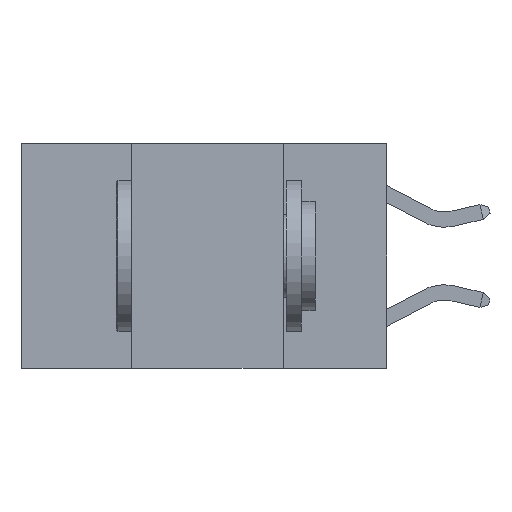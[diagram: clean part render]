
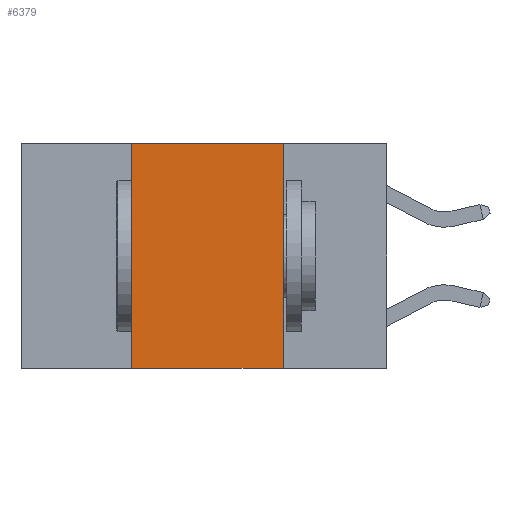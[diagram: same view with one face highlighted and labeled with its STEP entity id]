
A CAD part, left-side view. The second image highlights one B-rep face of the part: STEP entity #6379.
In plain terms, the highlighted planar face has unit normal (-1, 0, 0).
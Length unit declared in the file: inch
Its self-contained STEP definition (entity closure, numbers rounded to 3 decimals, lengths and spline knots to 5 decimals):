
#1246 = DIRECTION ( 'NONE',  ( 0., 0., 1. ) ) ;
#2895 = EDGE_CURVE ( 'NONE', #16272, #7749, #11159, .T. ) ;
#3063 = ORIENTED_EDGE ( 'NONE', *, *, #17406, .F. ) ;
#3518 = DIRECTION ( 'NONE',  ( 0., -1., 0. ) ) ;
#3544 = CARTESIAN_POINT ( 'NONE',  ( 0., 0.6, 0. ) ) ;
#4865 = VERTEX_POINT ( 'NONE', #10550 ) ;
#4994 = FACE_OUTER_BOUND ( 'NONE', #5014, .T. ) ;
#5014 = EDGE_LOOP ( 'NONE', ( #11372, #3063, #7511, #8008 ) ) ;
#5108 = EDGE_CURVE ( 'NONE', #4865, #9233, #6168, .T. ) ;
#5305 = CARTESIAN_POINT ( 'NONE',  ( 0., 0.17, 0. ) ) ;
#5511 = LINE ( 'NONE', #3544, #18115 ) ;
#5749 = VECTOR ( 'NONE', #3518, 39.37008 ) ;
#6168 = LINE ( 'NONE', #19264, #18697 ) ;
#6379 = ADVANCED_FACE ( 'NONE', ( #4994 ), #9672, .F. ) ;
#6440 = DIRECTION ( 'NONE',  ( 1., 0., 0. ) ) ;
#7029 = CARTESIAN_POINT ( 'NONE',  ( 0., 0.17, 0. ) ) ;
#7368 = EDGE_CURVE ( 'NONE', #4865, #7749, #10678, .T. ) ;
#7511 = ORIENTED_EDGE ( 'NONE', *, *, #5108, .F. ) ;
#7749 = VERTEX_POINT ( 'NONE', #17572 ) ;
#8008 = ORIENTED_EDGE ( 'NONE', *, *, #7368, .T. ) ;
#8591 = CARTESIAN_POINT ( 'NONE',  ( 0., 0.42, 0. ) ) ;
#9233 = VERTEX_POINT ( 'NONE', #8591 ) ;
#9672 = PLANE ( 'NONE',  #12310 ) ;
#10550 = CARTESIAN_POINT ( 'NONE',  ( 0., 0.42, -0.37 ) ) ;
#10678 = LINE ( 'NONE', #11780, #5749 ) ;
#11159 = LINE ( 'NONE', #5305, #18791 ) ;
#11341 = CARTESIAN_POINT ( 'NONE',  ( 0., 0.6, 0. ) ) ;
#11372 = ORIENTED_EDGE ( 'NONE', *, *, #2895, .F. ) ;
#11780 = CARTESIAN_POINT ( 'NONE',  ( 0., 0.6, -0.37 ) ) ;
#12310 = AXIS2_PLACEMENT_3D ( 'NONE', #11341, #6440, #17924 ) ;
#15228 = DIRECTION ( 'NONE',  ( 0., 0., -1. ) ) ;
#16272 = VERTEX_POINT ( 'NONE', #7029 ) ;
#16771 = DIRECTION ( 'NONE',  ( 0., -1., 0. ) ) ;
#17406 = EDGE_CURVE ( 'NONE', #9233, #16272, #5511, .T. ) ;
#17572 = CARTESIAN_POINT ( 'NONE',  ( 0., 0.17, -0.37 ) ) ;
#17924 = DIRECTION ( 'NONE',  ( 0., 0., -1. ) ) ;
#18115 = VECTOR ( 'NONE', #16771, 39.37008 ) ;
#18697 = VECTOR ( 'NONE', #1246, 39.37008 ) ;
#18791 = VECTOR ( 'NONE', #15228, 39.37008 ) ;
#19264 = CARTESIAN_POINT ( 'NONE',  ( 0., 0.42, 0. ) ) ;
